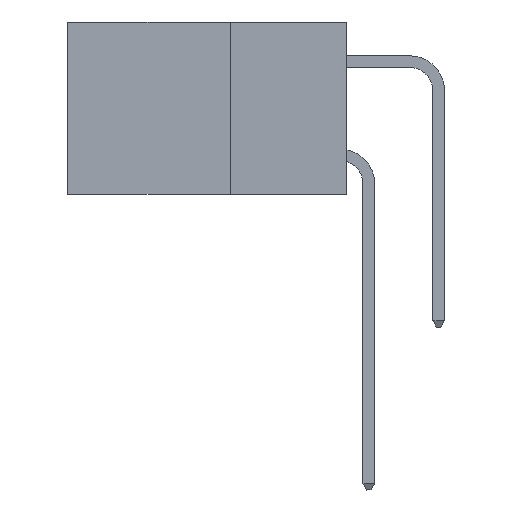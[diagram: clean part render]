
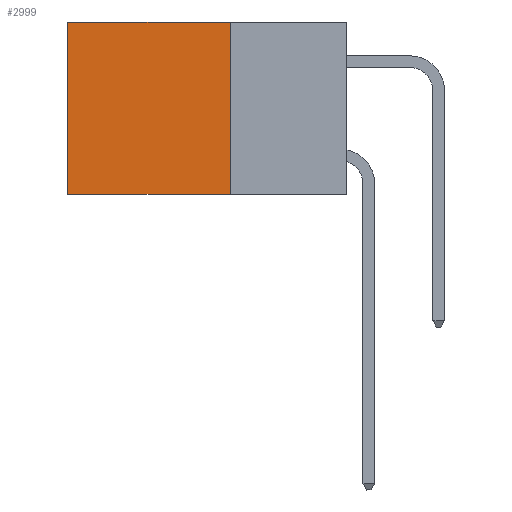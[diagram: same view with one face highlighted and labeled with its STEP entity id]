
A CAD part, left-side view. The second image highlights one B-rep face of the part: STEP entity #2999.
In plain terms, the highlighted planar face has unit normal (-1, 0, 0).
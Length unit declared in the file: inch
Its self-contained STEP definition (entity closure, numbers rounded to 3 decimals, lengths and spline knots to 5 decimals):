
#62 = VERTEX_POINT ( 'NONE', #11477 ) ;
#71 = EDGE_CURVE ( 'NONE', #16422, #19226, #3901, .T. ) ;
#1225 = LINE ( 'NONE', #23130, #22390 ) ;
#1716 = EDGE_CURVE ( 'NONE', #62, #9668, #19731, .T. ) ;
#1836 = DIRECTION ( 'NONE',  ( 0., 1., 0. ) ) ;
#1929 = ORIENTED_EDGE ( 'NONE', *, *, #71, .T. ) ;
#1994 = DIRECTION ( 'NONE',  ( 0., 0., -1. ) ) ;
#2999 = ADVANCED_FACE ( 'NONE', ( #21931 ), #12098, .F. ) ;
#3901 = LINE ( 'NONE', #26318, #15095 ) ;
#4408 = DIRECTION ( 'NONE',  ( 0., 1., 0. ) ) ;
#4894 = ORIENTED_EDGE ( 'NONE', *, *, #28200, .F. ) ;
#5737 = EDGE_LOOP ( 'NONE', ( #22721, #22309, #4894, #1929 ) ) ;
#6793 = LINE ( 'NONE', #17634, #24966 ) ;
#9479 = EDGE_CURVE ( 'NONE', #19226, #9668, #1225, .T. ) ;
#9668 = VERTEX_POINT ( 'NONE', #16897 ) ;
#11020 = CARTESIAN_POINT ( 'NONE',  ( 0.2875, 0.25, 0. ) ) ;
#11028 = AXIS2_PLACEMENT_3D ( 'NONE', #23038, #22825, #11242 ) ;
#11242 = DIRECTION ( 'NONE',  ( 0., 0., -1. ) ) ;
#11477 = CARTESIAN_POINT ( 'NONE',  ( 0.2875, 0.25, -0.37 ) ) ;
#12098 = PLANE ( 'NONE',  #11028 ) ;
#13053 = VECTOR ( 'NONE', #1836, 39.37008 ) ;
#15095 = VECTOR ( 'NONE', #4408, 39.37008 ) ;
#16422 = VERTEX_POINT ( 'NONE', #11020 ) ;
#16897 = CARTESIAN_POINT ( 'NONE',  ( 0.2875, 0.6, -0.37 ) ) ;
#17634 = CARTESIAN_POINT ( 'NONE',  ( 0.2875, 0.25, 0. ) ) ;
#19226 = VERTEX_POINT ( 'NONE', #27777 ) ;
#19731 = LINE ( 'NONE', #27785, #13053 ) ;
#21931 = FACE_OUTER_BOUND ( 'NONE', #5737, .T. ) ;
#22309 = ORIENTED_EDGE ( 'NONE', *, *, #1716, .F. ) ;
#22390 = VECTOR ( 'NONE', #1994, 39.37008 ) ;
#22721 = ORIENTED_EDGE ( 'NONE', *, *, #9479, .T. ) ;
#22825 = DIRECTION ( 'NONE',  ( 1., 0., 0. ) ) ;
#23038 = CARTESIAN_POINT ( 'NONE',  ( 0.2875, 0.25, 0. ) ) ;
#23130 = CARTESIAN_POINT ( 'NONE',  ( 0.2875, 0.6, 0. ) ) ;
#24966 = VECTOR ( 'NONE', #27176, 39.37008 ) ;
#26318 = CARTESIAN_POINT ( 'NONE',  ( 0.2875, 0.25, 0. ) ) ;
#27176 = DIRECTION ( 'NONE',  ( 0., 0., -1. ) ) ;
#27777 = CARTESIAN_POINT ( 'NONE',  ( 0.2875, 0.6, 0. ) ) ;
#27785 = CARTESIAN_POINT ( 'NONE',  ( 0.2875, 0.25, -0.37 ) ) ;
#28200 = EDGE_CURVE ( 'NONE', #16422, #62, #6793, .T. ) ;
